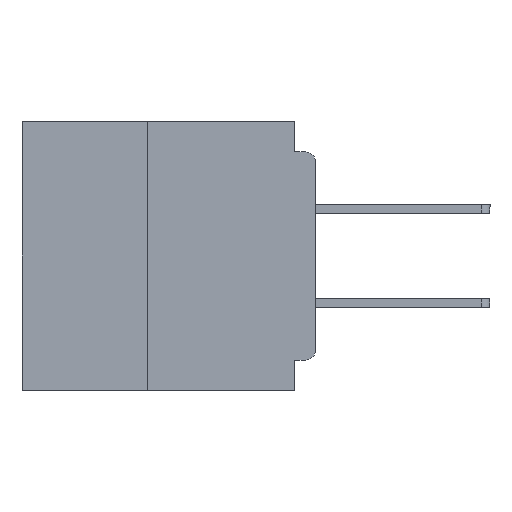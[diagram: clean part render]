
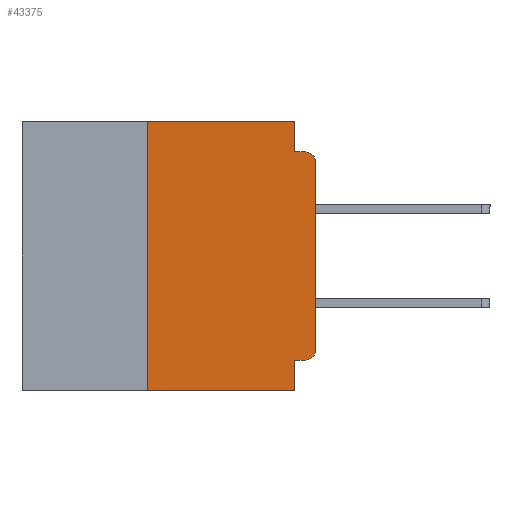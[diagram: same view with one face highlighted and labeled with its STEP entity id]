
A CAD part, left-side view. The second image highlights one B-rep face of the part: STEP entity #43375.
In plain terms, the highlighted planar face has unit normal (-1, 0, 0).
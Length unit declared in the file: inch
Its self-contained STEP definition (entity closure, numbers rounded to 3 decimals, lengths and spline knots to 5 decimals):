
#293 = ORIENTED_EDGE ( 'NONE', *, *, #41395, .T. ) ;
#684 = CARTESIAN_POINT ( 'NONE',  ( 0., 0.031, -0.355 ) ) ;
#959 = LINE ( 'NONE', #28534, #48628 ) ;
#2568 = ORIENTED_EDGE ( 'NONE', *, *, #39767, .F. ) ;
#3822 = EDGE_CURVE ( 'NONE', #19797, #26866, #25462, .T. ) ;
#4285 = VERTEX_POINT ( 'NONE', #39622 ) ;
#4415 = EDGE_LOOP ( 'NONE', ( #293, #19925, #34771, #2568, #31154, #47630, #13179, #44713, #5040, #48738 ) ) ;
#4906 = LINE ( 'NONE', #12311, #23689 ) ;
#5040 = ORIENTED_EDGE ( 'NONE', *, *, #25604, .F. ) ;
#6177 = AXIS2_PLACEMENT_3D ( 'NONE', #22297, #48509, #26045 ) ;
#6480 = CARTESIAN_POINT ( 'NONE',  ( 0., 0.25, 0. ) ) ;
#6696 = LINE ( 'NONE', #36210, #45399 ) ;
#7491 = VECTOR ( 'NONE', #36397, 39.37008 ) ;
#7802 = LINE ( 'NONE', #43776, #17828 ) ;
#8995 = DIRECTION ( 'NONE',  ( 0., 0., -1. ) ) ;
#9881 = DIRECTION ( 'NONE',  ( 0., 0., 1. ) ) ;
#10014 = DIRECTION ( 'NONE',  ( 0., 0., -1. ) ) ;
#10224 = CARTESIAN_POINT ( 'NONE',  ( 0., 0.031, -0.4 ) ) ;
#10795 = EDGE_CURVE ( 'NONE', #41803, #4285, #33785, .T. ) ;
#12311 = CARTESIAN_POINT ( 'NONE',  ( 0., 0., -0.355 ) ) ;
#12445 = VECTOR ( 'NONE', #24621, 39.37008 ) ;
#12978 = CARTESIAN_POINT ( 'NONE',  ( 0., 0.015, -0.34 ) ) ;
#13179 = ORIENTED_EDGE ( 'NONE', *, *, #34897, .T. ) ;
#13667 = AXIS2_PLACEMENT_3D ( 'NONE', #16410, #31378, #8995 ) ;
#13920 = VECTOR ( 'NONE', #27296, 39.37008 ) ;
#15204 = EDGE_CURVE ( 'NONE', #36220, #26866, #7802, .T. ) ;
#15748 = CARTESIAN_POINT ( 'NONE',  ( 0., 0., 0. ) ) ;
#16410 = CARTESIAN_POINT ( 'NONE',  ( 0., 0.437, 0. ) ) ;
#16750 = DIRECTION ( 'NONE',  ( 0., 0., -1. ) ) ;
#17828 = VECTOR ( 'NONE', #21311, 39.37008 ) ;
#19006 = EDGE_CURVE ( 'NONE', #35990, #34946, #46176, .T. ) ;
#19513 = DIRECTION ( 'NONE',  ( 0., 0., 1. ) ) ;
#19797 = VERTEX_POINT ( 'NONE', #37336 ) ;
#19925 = ORIENTED_EDGE ( 'NONE', *, *, #3822, .T. ) ;
#21311 = DIRECTION ( 'NONE',  ( 0., -1., 0. ) ) ;
#22297 = CARTESIAN_POINT ( 'NONE',  ( 0., 0.015, -0.06 ) ) ;
#23689 = VECTOR ( 'NONE', #42242, 39.37008 ) ;
#23866 = PLANE ( 'NONE',  #13667 ) ;
#23883 = FACE_OUTER_BOUND ( 'NONE', #4415, .T. ) ;
#24621 = DIRECTION ( 'NONE',  ( 0., -1., 0. ) ) ;
#24657 = VECTOR ( 'NONE', #19513, 39.37008 ) ;
#25462 = CIRCLE ( 'NONE', #6177, 0.015 ) ;
#25502 = VERTEX_POINT ( 'NONE', #37849 ) ;
#25604 = EDGE_CURVE ( 'NONE', #25502, #35990, #4906, .T. ) ;
#26045 = DIRECTION ( 'NONE',  ( 0., 0., -1. ) ) ;
#26806 = AXIS2_PLACEMENT_3D ( 'NONE', #12978, #39136, #16750 ) ;
#26866 = VERTEX_POINT ( 'NONE', #38000 ) ;
#27268 = CARTESIAN_POINT ( 'NONE',  ( 0., 0.25, -0.4 ) ) ;
#27296 = DIRECTION ( 'NONE',  ( 0., -1., 0. ) ) ;
#28403 = CARTESIAN_POINT ( 'NONE',  ( 0., 0.437, -0.4 ) ) ;
#28534 = CARTESIAN_POINT ( 'NONE',  ( 0., 0.25, -0.4 ) ) ;
#31154 = ORIENTED_EDGE ( 'NONE', *, *, #10795, .F. ) ;
#31378 = DIRECTION ( 'NONE',  ( 1., 0., 0. ) ) ;
#33785 = LINE ( 'NONE', #42217, #13920 ) ;
#34168 = EDGE_CURVE ( 'NONE', #25502, #47592, #36508, .T. ) ;
#34771 = ORIENTED_EDGE ( 'NONE', *, *, #15204, .F. ) ;
#34897 = EDGE_CURVE ( 'NONE', #44951, #34946, #42294, .T. ) ;
#34946 = VERTEX_POINT ( 'NONE', #43675 ) ;
#35834 = LINE ( 'NONE', #15748, #24657 ) ;
#35990 = VERTEX_POINT ( 'NONE', #684 ) ;
#36210 = CARTESIAN_POINT ( 'NONE',  ( 0., 0.031, 0. ) ) ;
#36220 = VERTEX_POINT ( 'NONE', #43631 ) ;
#36397 = DIRECTION ( 'NONE',  ( 0., 0., -1. ) ) ;
#36508 = CIRCLE ( 'NONE', #26806, 0.015 ) ;
#37336 = CARTESIAN_POINT ( 'NONE',  ( 0., 0., -0.06 ) ) ;
#37849 = CARTESIAN_POINT ( 'NONE',  ( 0., 0.015, -0.355 ) ) ;
#38000 = CARTESIAN_POINT ( 'NONE',  ( 0., 0.015, -0.045 ) ) ;
#39136 = DIRECTION ( 'NONE',  ( -1., 0., 0. ) ) ;
#39622 = CARTESIAN_POINT ( 'NONE',  ( 0., 0.031, 0. ) ) ;
#39767 = EDGE_CURVE ( 'NONE', #4285, #36220, #6696, .T. ) ;
#41395 = EDGE_CURVE ( 'NONE', #47592, #19797, #35834, .T. ) ;
#41803 = VERTEX_POINT ( 'NONE', #6480 ) ;
#42217 = CARTESIAN_POINT ( 'NONE',  ( 0., 0.437, 0. ) ) ;
#42242 = DIRECTION ( 'NONE',  ( 0., 1., 0. ) ) ;
#42294 = LINE ( 'NONE', #28403, #12445 ) ;
#42358 = EDGE_CURVE ( 'NONE', #44951, #41803, #959, .T. ) ;
#43375 = ADVANCED_FACE ( 'NONE', ( #23883 ), #23866, .F. ) ;
#43631 = CARTESIAN_POINT ( 'NONE',  ( 0., 0.031, -0.045 ) ) ;
#43675 = CARTESIAN_POINT ( 'NONE',  ( 0., 0.031, -0.4 ) ) ;
#43776 = CARTESIAN_POINT ( 'NONE',  ( 0., 0., -0.045 ) ) ;
#44713 = ORIENTED_EDGE ( 'NONE', *, *, #19006, .F. ) ;
#44951 = VERTEX_POINT ( 'NONE', #27268 ) ;
#45399 = VECTOR ( 'NONE', #10014, 39.37008 ) ;
#46176 = LINE ( 'NONE', #10224, #7491 ) ;
#46360 = CARTESIAN_POINT ( 'NONE',  ( 0., 0., -0.34 ) ) ;
#47592 = VERTEX_POINT ( 'NONE', #46360 ) ;
#47630 = ORIENTED_EDGE ( 'NONE', *, *, #42358, .F. ) ;
#48509 = DIRECTION ( 'NONE',  ( -1., 0., 0. ) ) ;
#48628 = VECTOR ( 'NONE', #9881, 39.37008 ) ;
#48738 = ORIENTED_EDGE ( 'NONE', *, *, #34168, .T. ) ;
